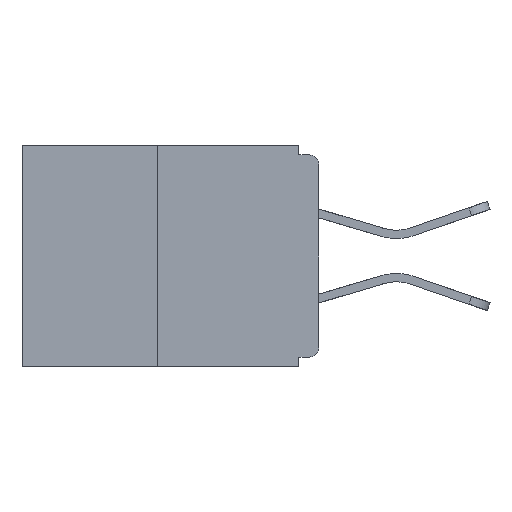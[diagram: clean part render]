
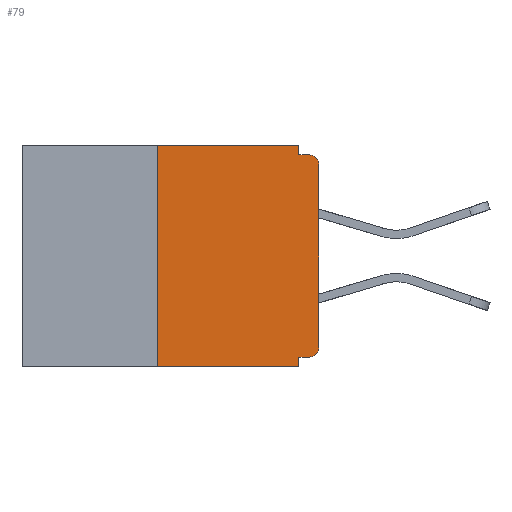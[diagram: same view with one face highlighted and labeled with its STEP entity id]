
A CAD part, left-side view. The second image highlights one B-rep face of the part: STEP entity #79.
In plain terms, the highlighted planar face has unit normal (-1, 0, 0).
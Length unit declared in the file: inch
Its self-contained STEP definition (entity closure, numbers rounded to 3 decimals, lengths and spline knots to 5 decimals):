
#79 = ADVANCED_FACE ( 'NONE', ( #12153 ), #11154, .F. ) ;
#165 = EDGE_LOOP ( 'NONE', ( #21060, #7981, #3213, #1301, #8654, #3148, #16820, #19395, #8617, #22376 ) ) ;
#465 = VECTOR ( 'NONE', #16742, 39.37008 ) ;
#592 = VECTOR ( 'NONE', #15923, 39.37008 ) ;
#694 = DIRECTION ( 'NONE',  ( 1., 0., 0. ) ) ;
#1056 = CARTESIAN_POINT ( 'NONE',  ( 0., 0.031, -0.015 ) ) ;
#1301 = ORIENTED_EDGE ( 'NONE', *, *, #13298, .F. ) ;
#1546 = LINE ( 'NONE', #16892, #465 ) ;
#1553 = AXIS2_PLACEMENT_3D ( 'NONE', #3934, #19353, #12573 ) ;
#1688 = VECTOR ( 'NONE', #16231, 39.37008 ) ;
#2177 = EDGE_CURVE ( 'NONE', #12487, #16419, #7293, .T. ) ;
#2310 = VECTOR ( 'NONE', #11714, 39.37008 ) ;
#2837 = EDGE_CURVE ( 'NONE', #8139, #13046, #5656, .T. ) ;
#2946 = DIRECTION ( 'NONE',  ( 0., -1., 0. ) ) ;
#3053 = CARTESIAN_POINT ( 'NONE',  ( 0., 0.015, -0.015 ) ) ;
#3148 = ORIENTED_EDGE ( 'NONE', *, *, #2177, .T. ) ;
#3213 = ORIENTED_EDGE ( 'NONE', *, *, #5781, .T. ) ;
#3602 = VERTEX_POINT ( 'NONE', #19340 ) ;
#3934 = CARTESIAN_POINT ( 'NONE',  ( 0., 0.015, -0.313 ) ) ;
#4184 = LINE ( 'NONE', #6487, #21008 ) ;
#4251 = CARTESIAN_POINT ( 'NONE',  ( 0., 0., -0.313 ) ) ;
#4285 = EDGE_CURVE ( 'NONE', #16419, #21822, #10755, .T. ) ;
#4373 = CIRCLE ( 'NONE', #20361, 0.015 ) ;
#5173 = EDGE_CURVE ( 'NONE', #13710, #12707, #18328, .T. ) ;
#5501 = VECTOR ( 'NONE', #11190, 39.37008 ) ;
#5593 = EDGE_CURVE ( 'NONE', #13046, #13710, #9328, .T. ) ;
#5656 = LINE ( 'NONE', #18238, #8932 ) ;
#5781 = EDGE_CURVE ( 'NONE', #8139, #3602, #11243, .T. ) ;
#6464 = CARTESIAN_POINT ( 'NONE',  ( 0., 0., 0. ) ) ;
#6487 = CARTESIAN_POINT ( 'NONE',  ( 0., 0., -0.015 ) ) ;
#7293 = CIRCLE ( 'NONE', #1553, 0.015 ) ;
#7385 = CARTESIAN_POINT ( 'NONE',  ( 0., 0.46, -0.343 ) ) ;
#7568 = DIRECTION ( 'NONE',  ( 0., 0., 1. ) ) ;
#7981 = ORIENTED_EDGE ( 'NONE', *, *, #2837, .F. ) ;
#8139 = VERTEX_POINT ( 'NONE', #21546 ) ;
#8273 = DIRECTION ( 'NONE',  ( 0., 0., -1. ) ) ;
#8617 = ORIENTED_EDGE ( 'NONE', *, *, #17892, .F. ) ;
#8654 = ORIENTED_EDGE ( 'NONE', *, *, #10274, .F. ) ;
#8932 = VECTOR ( 'NONE', #7568, 39.37008 ) ;
#9328 = LINE ( 'NONE', #10559, #592 ) ;
#9480 = CARTESIAN_POINT ( 'NONE',  ( 0., 0.46, 0. ) ) ;
#9967 = CARTESIAN_POINT ( 'NONE',  ( 0., 0.031, 0. ) ) ;
#10126 = LINE ( 'NONE', #11476, #5501 ) ;
#10180 = CARTESIAN_POINT ( 'NONE',  ( 0., 0.031, 0. ) ) ;
#10215 = DIRECTION ( 'NONE',  ( -1., 0., 0. ) ) ;
#10274 = EDGE_CURVE ( 'NONE', #12487, #18399, #10126, .T. ) ;
#10559 = CARTESIAN_POINT ( 'NONE',  ( 0., 0.46, 0. ) ) ;
#10755 = LINE ( 'NONE', #6464, #2310 ) ;
#11154 = PLANE ( 'NONE',  #16374 ) ;
#11190 = DIRECTION ( 'NONE',  ( 0., 1., 0. ) ) ;
#11243 = LINE ( 'NONE', #7385, #1688 ) ;
#11476 = CARTESIAN_POINT ( 'NONE',  ( 0., 0., -0.328 ) ) ;
#11714 = DIRECTION ( 'NONE',  ( 0., 0., 1. ) ) ;
#12153 = FACE_OUTER_BOUND ( 'NONE', #165, .T. ) ;
#12388 = CARTESIAN_POINT ( 'NONE',  ( 0., 0.031, -0.328 ) ) ;
#12487 = VERTEX_POINT ( 'NONE', #14560 ) ;
#12573 = DIRECTION ( 'NONE',  ( 0., 0., -1. ) ) ;
#12707 = VERTEX_POINT ( 'NONE', #1056 ) ;
#12870 = VERTEX_POINT ( 'NONE', #3053 ) ;
#13046 = VERTEX_POINT ( 'NONE', #17072 ) ;
#13298 = EDGE_CURVE ( 'NONE', #18399, #3602, #1546, .T. ) ;
#13710 = VERTEX_POINT ( 'NONE', #10180 ) ;
#14560 = CARTESIAN_POINT ( 'NONE',  ( 0., 0.015, -0.328 ) ) ;
#14766 = EDGE_CURVE ( 'NONE', #21822, #12870, #4373, .T. ) ;
#15923 = DIRECTION ( 'NONE',  ( 0., -1., 0. ) ) ;
#16231 = DIRECTION ( 'NONE',  ( 0., -1., 0. ) ) ;
#16299 = CARTESIAN_POINT ( 'NONE',  ( 0., 0., -0.03 ) ) ;
#16374 = AXIS2_PLACEMENT_3D ( 'NONE', #9480, #694, #18195 ) ;
#16419 = VERTEX_POINT ( 'NONE', #4251 ) ;
#16742 = DIRECTION ( 'NONE',  ( 0., 0., -1. ) ) ;
#16820 = ORIENTED_EDGE ( 'NONE', *, *, #4285, .T. ) ;
#16892 = CARTESIAN_POINT ( 'NONE',  ( 0., 0.031, -0.343 ) ) ;
#17072 = CARTESIAN_POINT ( 'NONE',  ( 0., 0.25, 0. ) ) ;
#17892 = EDGE_CURVE ( 'NONE', #12707, #12870, #4184, .T. ) ;
#18195 = DIRECTION ( 'NONE',  ( 0., 0., -1. ) ) ;
#18238 = CARTESIAN_POINT ( 'NONE',  ( 0., 0.25, 0. ) ) ;
#18328 = LINE ( 'NONE', #9967, #18851 ) ;
#18399 = VERTEX_POINT ( 'NONE', #12388 ) ;
#18851 = VECTOR ( 'NONE', #8273, 39.37008 ) ;
#19340 = CARTESIAN_POINT ( 'NONE',  ( 0., 0.031, -0.343 ) ) ;
#19353 = DIRECTION ( 'NONE',  ( -1., 0., 0. ) ) ;
#19395 = ORIENTED_EDGE ( 'NONE', *, *, #14766, .T. ) ;
#20361 = AXIS2_PLACEMENT_3D ( 'NONE', #20585, #10215, #22291 ) ;
#20585 = CARTESIAN_POINT ( 'NONE',  ( 0., 0.015, -0.03 ) ) ;
#21008 = VECTOR ( 'NONE', #2946, 39.37008 ) ;
#21060 = ORIENTED_EDGE ( 'NONE', *, *, #5593, .F. ) ;
#21546 = CARTESIAN_POINT ( 'NONE',  ( 0., 0.25, -0.343 ) ) ;
#21822 = VERTEX_POINT ( 'NONE', #16299 ) ;
#22291 = DIRECTION ( 'NONE',  ( 0., 0., -1. ) ) ;
#22376 = ORIENTED_EDGE ( 'NONE', *, *, #5173, .F. ) ;
